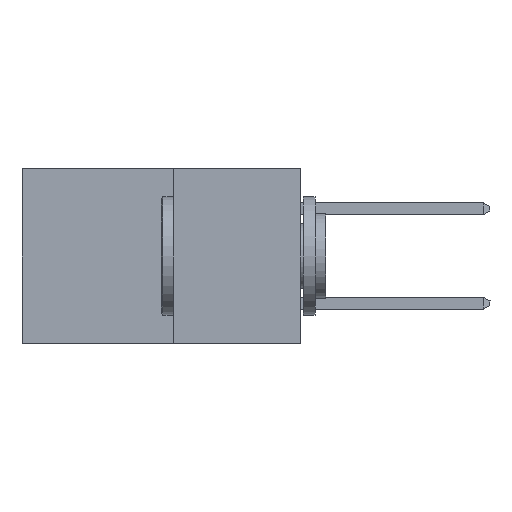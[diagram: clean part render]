
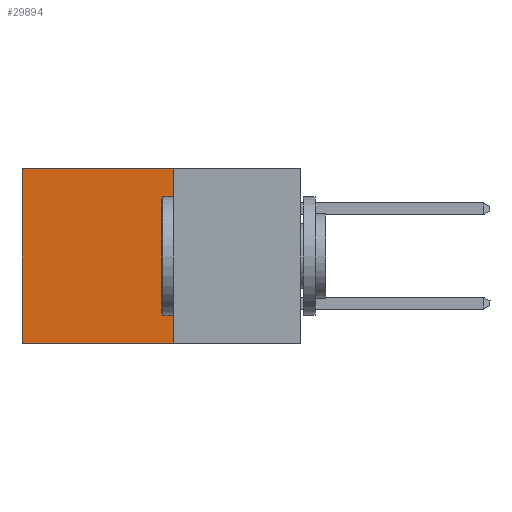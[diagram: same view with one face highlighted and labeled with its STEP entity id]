
A CAD part, left-side view. The second image highlights one B-rep face of the part: STEP entity #29894.
In plain terms, the highlighted planar face has unit normal (-1, 0, 0).
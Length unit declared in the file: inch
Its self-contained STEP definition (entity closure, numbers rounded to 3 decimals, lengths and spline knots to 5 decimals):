
#797 = VERTEX_POINT ( 'NONE', #30408 ) ;
#2899 = ORIENTED_EDGE ( 'NONE', *, *, #33030, .T. ) ;
#3453 = CARTESIAN_POINT ( 'NONE',  ( 0.277, 0.59, 0. ) ) ;
#3688 = VERTEX_POINT ( 'NONE', #6367 ) ;
#4033 = VECTOR ( 'NONE', #14133, 39.37008 ) ;
#4597 = ORIENTED_EDGE ( 'NONE', *, *, #28534, .F. ) ;
#4818 = CARTESIAN_POINT ( 'NONE',  ( 0.277, 0.27, -0.37 ) ) ;
#6367 = CARTESIAN_POINT ( 'NONE',  ( 0.277, 0.27, 0. ) ) ;
#7338 = AXIS2_PLACEMENT_3D ( 'NONE', #4818, #29396, #13111 ) ;
#7593 = PLANE ( 'NONE',  #7338 ) ;
#7770 = VERTEX_POINT ( 'NONE', #3453 ) ;
#7841 = ORIENTED_EDGE ( 'NONE', *, *, #19283, .T. ) ;
#10145 = LINE ( 'NONE', #14083, #16511 ) ;
#10585 = DIRECTION ( 'NONE',  ( 0., 0., -1. ) ) ;
#10685 = DIRECTION ( 'NONE',  ( 0., 1., 0. ) ) ;
#11397 = LINE ( 'NONE', #32967, #4033 ) ;
#13111 = DIRECTION ( 'NONE',  ( 0., 0., -1. ) ) ;
#14083 = CARTESIAN_POINT ( 'NONE',  ( 0.277, 0.59, -0.37 ) ) ;
#14133 = DIRECTION ( 'NONE',  ( 0., 1., 0. ) ) ;
#16511 = VECTOR ( 'NONE', #16797, 39.37008 ) ;
#16797 = DIRECTION ( 'NONE',  ( 0., 0., -1. ) ) ;
#16828 = VECTOR ( 'NONE', #10685, 39.37008 ) ;
#17418 = FACE_OUTER_BOUND ( 'NONE', #33995, .T. ) ;
#18157 = VECTOR ( 'NONE', #10585, 39.37008 ) ;
#19283 = EDGE_CURVE ( 'NONE', #7770, #797, #10145, .T. ) ;
#22201 = CARTESIAN_POINT ( 'NONE',  ( 0.277, 0.27, -0.37 ) ) ;
#24055 = LINE ( 'NONE', #26962, #16828 ) ;
#25409 = LINE ( 'NONE', #34849, #18157 ) ;
#25592 = VERTEX_POINT ( 'NONE', #22201 ) ;
#26962 = CARTESIAN_POINT ( 'NONE',  ( 0.277, 0.27, 0. ) ) ;
#28534 = EDGE_CURVE ( 'NONE', #3688, #25592, #25409, .T. ) ;
#28776 = EDGE_CURVE ( 'NONE', #25592, #797, #11397, .T. ) ;
#29354 = ORIENTED_EDGE ( 'NONE', *, *, #28776, .F. ) ;
#29396 = DIRECTION ( 'NONE',  ( 1., 0., 0. ) ) ;
#29894 = ADVANCED_FACE ( 'NONE', ( #17418 ), #7593, .F. ) ;
#30408 = CARTESIAN_POINT ( 'NONE',  ( 0.277, 0.59, -0.37 ) ) ;
#32967 = CARTESIAN_POINT ( 'NONE',  ( 0.277, 0.27, -0.37 ) ) ;
#33030 = EDGE_CURVE ( 'NONE', #3688, #7770, #24055, .T. ) ;
#33995 = EDGE_LOOP ( 'NONE', ( #7841, #29354, #4597, #2899 ) ) ;
#34849 = CARTESIAN_POINT ( 'NONE',  ( 0.277, 0.27, -0.37 ) ) ;
